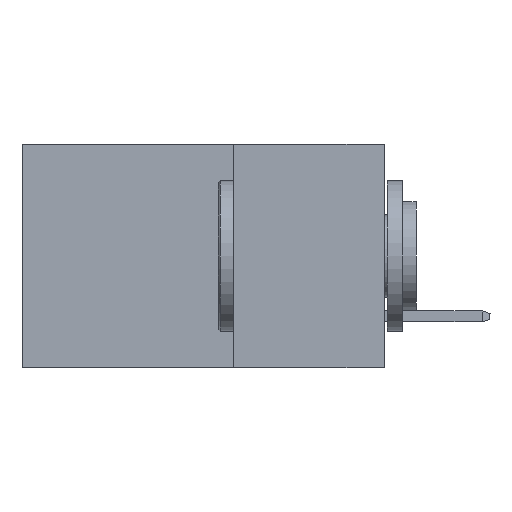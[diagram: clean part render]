
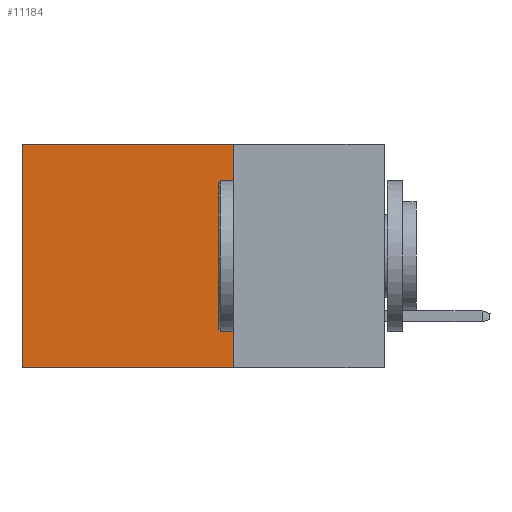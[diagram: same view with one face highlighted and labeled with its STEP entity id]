
A CAD part, left-side view. The second image highlights one B-rep face of the part: STEP entity #11184.
In plain terms, the highlighted planar face has unit normal (-1, 0, 0).
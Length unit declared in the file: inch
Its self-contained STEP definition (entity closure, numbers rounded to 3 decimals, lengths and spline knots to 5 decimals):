
#440 = EDGE_CURVE ( 'NONE', #5954, #2765, #19192, .T. ) ;
#639 = EDGE_CURVE ( 'NONE', #12918, #2765, #8032, .T. ) ;
#1326 = ORIENTED_EDGE ( 'NONE', *, *, #639, .T. ) ;
#1611 = CARTESIAN_POINT ( 'NONE',  ( 0.298, 0.25, -0.37 ) ) ;
#2040 = CARTESIAN_POINT ( 'NONE',  ( 0.298, 0.25, 0. ) ) ;
#2375 = ORIENTED_EDGE ( 'NONE', *, *, #15797, .T. ) ;
#2765 = VERTEX_POINT ( 'NONE', #7743 ) ;
#3238 = VECTOR ( 'NONE', #9286, 39.37008 ) ;
#4018 = EDGE_LOOP ( 'NONE', ( #1326, #4600, #11794, #2375 ) ) ;
#4312 = CARTESIAN_POINT ( 'NONE',  ( 0.298, 0.25, 0. ) ) ;
#4600 = ORIENTED_EDGE ( 'NONE', *, *, #440, .F. ) ;
#5067 = AXIS2_PLACEMENT_3D ( 'NONE', #2040, #6689, #17982 ) ;
#5954 = VERTEX_POINT ( 'NONE', #1611 ) ;
#6298 = VECTOR ( 'NONE', #9929, 39.37008 ) ;
#6689 = DIRECTION ( 'NONE',  ( 1., 0., 0. ) ) ;
#7743 = CARTESIAN_POINT ( 'NONE',  ( 0.298, 0.6, -0.37 ) ) ;
#7944 = EDGE_CURVE ( 'NONE', #11631, #5954, #16849, .T. ) ;
#8032 = LINE ( 'NONE', #19600, #6298 ) ;
#9286 = DIRECTION ( 'NONE',  ( 0., 0., -1. ) ) ;
#9929 = DIRECTION ( 'NONE',  ( 0., 0., -1. ) ) ;
#11096 = CARTESIAN_POINT ( 'NONE',  ( 0.298, 0.25, 0. ) ) ;
#11184 = ADVANCED_FACE ( 'NONE', ( #11956 ), #13305, .F. ) ;
#11328 = DIRECTION ( 'NONE',  ( 0., 1., 0. ) ) ;
#11631 = VERTEX_POINT ( 'NONE', #11096 ) ;
#11794 = ORIENTED_EDGE ( 'NONE', *, *, #7944, .F. ) ;
#11956 = FACE_OUTER_BOUND ( 'NONE', #4018, .T. ) ;
#12918 = VERTEX_POINT ( 'NONE', #20285 ) ;
#13305 = PLANE ( 'NONE',  #5067 ) ;
#13865 = VECTOR ( 'NONE', #11328, 39.37008 ) ;
#14196 = VECTOR ( 'NONE', #20364, 39.37008 ) ;
#15797 = EDGE_CURVE ( 'NONE', #11631, #12918, #19244, .T. ) ;
#16849 = LINE ( 'NONE', #17337, #3238 ) ;
#17337 = CARTESIAN_POINT ( 'NONE',  ( 0.298, 0.25, 0. ) ) ;
#17982 = DIRECTION ( 'NONE',  ( 0., 0., -1. ) ) ;
#19192 = LINE ( 'NONE', #20853, #13865 ) ;
#19244 = LINE ( 'NONE', #4312, #14196 ) ;
#19600 = CARTESIAN_POINT ( 'NONE',  ( 0.298, 0.6, 0. ) ) ;
#20285 = CARTESIAN_POINT ( 'NONE',  ( 0.298, 0.6, 0. ) ) ;
#20364 = DIRECTION ( 'NONE',  ( 0., 1., 0. ) ) ;
#20853 = CARTESIAN_POINT ( 'NONE',  ( 0.298, 0.25, -0.37 ) ) ;
